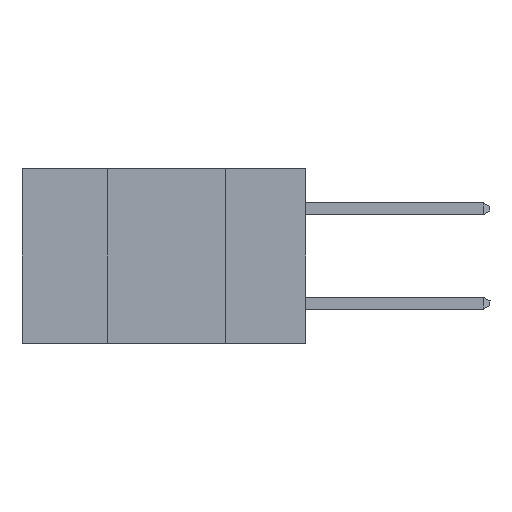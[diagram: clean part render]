
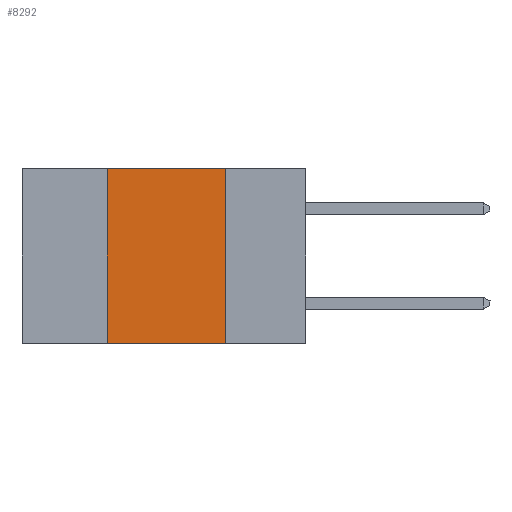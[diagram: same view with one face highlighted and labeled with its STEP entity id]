
A CAD part, left-side view. The second image highlights one B-rep face of the part: STEP entity #8292.
In plain terms, the highlighted planar face has unit normal (-1, 0, 0).
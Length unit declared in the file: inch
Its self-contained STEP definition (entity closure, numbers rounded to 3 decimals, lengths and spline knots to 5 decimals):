
#252 = DIRECTION ( 'NONE',  ( 0., -1., 0. ) ) ;
#1576 = VECTOR ( 'NONE', #12957, 39.37008 ) ;
#1680 = CARTESIAN_POINT ( 'NONE',  ( 0., 0.42, 0. ) ) ;
#3712 = ORIENTED_EDGE ( 'NONE', *, *, #9066, .F. ) ;
#4185 = CARTESIAN_POINT ( 'NONE',  ( 0., 0.6, 0. ) ) ;
#4281 = VERTEX_POINT ( 'NONE', #16608 ) ;
#4348 = EDGE_CURVE ( 'NONE', #23414, #4868, #20955, .T. ) ;
#4868 = VERTEX_POINT ( 'NONE', #8721 ) ;
#6136 = DIRECTION ( 'NONE',  ( 0., 0., -1. ) ) ;
#7121 = CARTESIAN_POINT ( 'NONE',  ( 0., 0.42, -0.37 ) ) ;
#8292 = ADVANCED_FACE ( 'NONE', ( #22639 ), #11895, .F. ) ;
#8681 = ORIENTED_EDGE ( 'NONE', *, *, #14218, .T. ) ;
#8721 = CARTESIAN_POINT ( 'NONE',  ( 0., 0.17, 0. ) ) ;
#9066 = EDGE_CURVE ( 'NONE', #4868, #23658, #15497, .T. ) ;
#9161 = DIRECTION ( 'NONE',  ( 0., -1., 0. ) ) ;
#9221 = EDGE_CURVE ( 'NONE', #4281, #23414, #22013, .T. ) ;
#10414 = VECTOR ( 'NONE', #14462, 39.37008 ) ;
#11395 = EDGE_LOOP ( 'NONE', ( #3712, #13472, #19718, #8681 ) ) ;
#11895 = PLANE ( 'NONE',  #20356 ) ;
#12957 = DIRECTION ( 'NONE',  ( 0., 0., 1. ) ) ;
#13472 = ORIENTED_EDGE ( 'NONE', *, *, #4348, .F. ) ;
#13788 = CARTESIAN_POINT ( 'NONE',  ( 0., 0.6, -0.37 ) ) ;
#14218 = EDGE_CURVE ( 'NONE', #4281, #23658, #18483, .T. ) ;
#14462 = DIRECTION ( 'NONE',  ( 0., 0., -1. ) ) ;
#15497 = LINE ( 'NONE', #22009, #10414 ) ;
#16608 = CARTESIAN_POINT ( 'NONE',  ( 0., 0.42, -0.37 ) ) ;
#17624 = DIRECTION ( 'NONE',  ( 1., 0., 0. ) ) ;
#17739 = CARTESIAN_POINT ( 'NONE',  ( 0., 0.17, -0.37 ) ) ;
#18483 = LINE ( 'NONE', #13788, #23505 ) ;
#19718 = ORIENTED_EDGE ( 'NONE', *, *, #9221, .F. ) ;
#20356 = AXIS2_PLACEMENT_3D ( 'NONE', #4185, #17624, #6136 ) ;
#20955 = LINE ( 'NONE', #24283, #24761 ) ;
#22009 = CARTESIAN_POINT ( 'NONE',  ( 0., 0.17, -0.37 ) ) ;
#22013 = LINE ( 'NONE', #7121, #1576 ) ;
#22639 = FACE_OUTER_BOUND ( 'NONE', #11395, .T. ) ;
#23414 = VERTEX_POINT ( 'NONE', #1680 ) ;
#23505 = VECTOR ( 'NONE', #252, 39.37008 ) ;
#23658 = VERTEX_POINT ( 'NONE', #17739 ) ;
#24283 = CARTESIAN_POINT ( 'NONE',  ( 0., 0.6, 0. ) ) ;
#24761 = VECTOR ( 'NONE', #9161, 39.37008 ) ;
